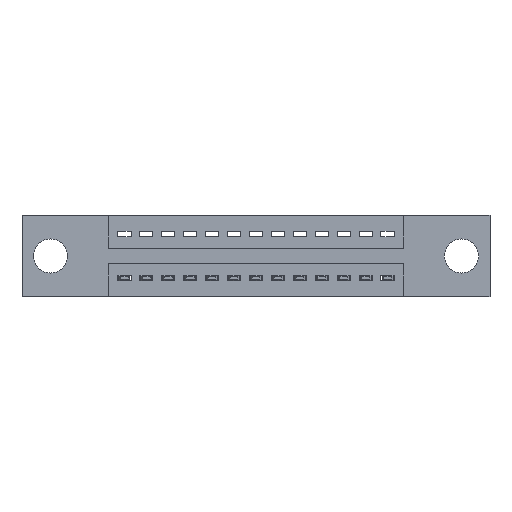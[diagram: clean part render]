
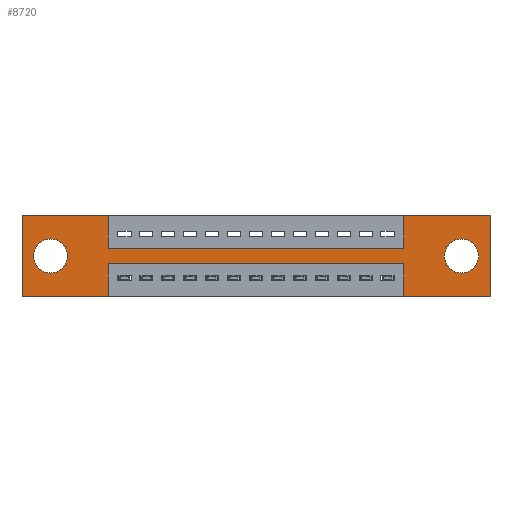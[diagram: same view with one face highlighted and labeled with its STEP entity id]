
A CAD part, front view. The second image highlights one B-rep face of the part: STEP entity #8720.
In plain terms, the highlighted planar face has unit normal (0, -1, 0).
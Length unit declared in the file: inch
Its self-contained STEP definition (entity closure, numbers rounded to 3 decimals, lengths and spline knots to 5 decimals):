
#270 = DIRECTION ( 'NONE',  ( 1., 0., 0. ) ) ;
#277 = VECTOR ( 'NONE', #8580, 39.37008 ) ;
#346 = VERTEX_POINT ( 'NONE', #3894 ) ;
#348 = LINE ( 'NONE', #9882, #1293 ) ;
#350 = CARTESIAN_POINT ( 'NONE',  ( 0.3925, 0., -0.15 ) ) ;
#443 = VERTEX_POINT ( 'NONE', #10243 ) ;
#567 = LINE ( 'NONE', #12195, #5150 ) ;
#646 = VERTEX_POINT ( 'NONE', #5089 ) ;
#901 = CARTESIAN_POINT ( 'NONE',  ( 0.13, 0., -0.107 ) ) ;
#906 = EDGE_CURVE ( 'NONE', #5767, #5690, #348, .T. ) ;
#951 = CARTESIAN_POINT ( 'NONE',  ( 1.7425, 0., -0.37 ) ) ;
#990 = EDGE_CURVE ( 'NONE', #11769, #11636, #4753, .T. ) ;
#1047 = VECTOR ( 'NONE', #12163, 39.37008 ) ;
#1293 = VECTOR ( 'NONE', #1474, 39.37008 ) ;
#1382 = ORIENTED_EDGE ( 'NONE', *, *, #9302, .F. ) ;
#1431 = VERTEX_POINT ( 'NONE', #7428 ) ;
#1454 = VECTOR ( 'NONE', #2695, 39.37008 ) ;
#1474 = DIRECTION ( 'NONE',  ( -1., 0., 0. ) ) ;
#1801 = CARTESIAN_POINT ( 'NONE',  ( 0., 0., -0.37 ) ) ;
#2099 = ORIENTED_EDGE ( 'NONE', *, *, #8531, .T. ) ;
#2127 = ORIENTED_EDGE ( 'NONE', *, *, #5831, .F. ) ;
#2137 = EDGE_CURVE ( 'NONE', #8384, #13415, #567, .T. ) ;
#2385 = FACE_BOUND ( 'NONE', #7747, .T. ) ;
#2518 = LINE ( 'NONE', #8944, #1047 ) ;
#2521 = DIRECTION ( 'NONE',  ( 0., 0., -1. ) ) ;
#2695 = DIRECTION ( 'NONE',  ( 1., 0., 0. ) ) ;
#2714 = VECTOR ( 'NONE', #2521, 39.37008 ) ;
#2877 = LINE ( 'NONE', #9422, #12211 ) ;
#2994 = EDGE_CURVE ( 'NONE', #346, #7902, #2518, .T. ) ;
#3264 = AXIS2_PLACEMENT_3D ( 'NONE', #3440, #4642, #7961 ) ;
#3434 = CARTESIAN_POINT ( 'NONE',  ( 0.3925, 0., 0. ) ) ;
#3440 = CARTESIAN_POINT ( 'NONE',  ( 0., 0., -0.37 ) ) ;
#3488 = ORIENTED_EDGE ( 'NONE', *, *, #11981, .F. ) ;
#3631 = LINE ( 'NONE', #12216, #13633 ) ;
#3663 = VERTEX_POINT ( 'NONE', #12548 ) ;
#3713 = LINE ( 'NONE', #3907, #5990 ) ;
#3721 = CARTESIAN_POINT ( 'NONE',  ( 0.3925, 0., -0.37 ) ) ;
#3894 = CARTESIAN_POINT ( 'NONE',  ( 0., 0., -0.37 ) ) ;
#3907 = CARTESIAN_POINT ( 'NONE',  ( 2.135, 0., 0. ) ) ;
#3952 = AXIS2_PLACEMENT_3D ( 'NONE', #13821, #10790, #12832 ) ;
#4342 = EDGE_CURVE ( 'NONE', #8558, #443, #12095, .T. ) ;
#4457 = CARTESIAN_POINT ( 'NONE',  ( 0., 0., 0. ) ) ;
#4642 = DIRECTION ( 'NONE',  ( 0., -1., 0. ) ) ;
#4753 = CIRCLE ( 'NONE', #10372, 0.078 ) ;
#4829 = CARTESIAN_POINT ( 'NONE',  ( 2.005, 0., -0.185 ) ) ;
#4844 = ORIENTED_EDGE ( 'NONE', *, *, #7290, .F. ) ;
#4914 = ORIENTED_EDGE ( 'NONE', *, *, #990, .T. ) ;
#4940 = CARTESIAN_POINT ( 'NONE',  ( 0.13, 0., -0.185 ) ) ;
#5089 = CARTESIAN_POINT ( 'NONE',  ( 1.7425, 0., -0.22 ) ) ;
#5150 = VECTOR ( 'NONE', #8906, 39.37008 ) ;
#5632 = FACE_OUTER_BOUND ( 'NONE', #6299, .T. ) ;
#5690 = VERTEX_POINT ( 'NONE', #6253 ) ;
#5699 = EDGE_CURVE ( 'NONE', #3663, #1431, #2877, .T. ) ;
#5767 = VERTEX_POINT ( 'NONE', #12012 ) ;
#5794 = VECTOR ( 'NONE', #8311, 39.37008 ) ;
#5831 = EDGE_CURVE ( 'NONE', #646, #8558, #8516, .T. ) ;
#5882 = ORIENTED_EDGE ( 'NONE', *, *, #12371, .T. ) ;
#5990 = VECTOR ( 'NONE', #8092, 39.37008 ) ;
#5998 = CIRCLE ( 'NONE', #3952, 0.078 ) ;
#6052 = DIRECTION ( 'NONE',  ( -1., 0., 0. ) ) ;
#6253 = CARTESIAN_POINT ( 'NONE',  ( 1.7425, 0., -0.37 ) ) ;
#6299 = EDGE_LOOP ( 'NONE', ( #13230, #2127, #3488, #9588, #1382, #6541, #6807, #11499, #13559, #11309, #10766, #4844 ) ) ;
#6483 = CARTESIAN_POINT ( 'NONE',  ( 0.13, 0., -0.263 ) ) ;
#6541 = ORIENTED_EDGE ( 'NONE', *, *, #5699, .F. ) ;
#6593 = CARTESIAN_POINT ( 'NONE',  ( 0.3925, 0., -0.22 ) ) ;
#6807 = ORIENTED_EDGE ( 'NONE', *, *, #10919, .F. ) ;
#6870 = DIRECTION ( 'NONE',  ( 0., 0., 1. ) ) ;
#6879 = CIRCLE ( 'NONE', #12029, 0.078 ) ;
#6924 = AXIS2_PLACEMENT_3D ( 'NONE', #4829, #11451, #10260 ) ;
#7190 = LINE ( 'NONE', #951, #5794 ) ;
#7290 = EDGE_CURVE ( 'NONE', #443, #346, #8429, .T. ) ;
#7428 = CARTESIAN_POINT ( 'NONE',  ( 2.135, 0., 0. ) ) ;
#7747 = EDGE_LOOP ( 'NONE', ( #5882, #4914 ) ) ;
#7817 = EDGE_LOOP ( 'NONE', ( #9727, #2099 ) ) ;
#7902 = VERTEX_POINT ( 'NONE', #4457 ) ;
#7961 = DIRECTION ( 'NONE',  ( 0., 0., -1. ) ) ;
#8046 = VECTOR ( 'NONE', #270, 39.37008 ) ;
#8092 = DIRECTION ( 'NONE',  ( 0., 0., -1. ) ) ;
#8311 = DIRECTION ( 'NONE',  ( 0., 0., 1. ) ) ;
#8384 = VERTEX_POINT ( 'NONE', #3434 ) ;
#8429 = LINE ( 'NONE', #1801, #9529 ) ;
#8516 = LINE ( 'NONE', #6593, #277 ) ;
#8531 = EDGE_CURVE ( 'NONE', #11574, #11751, #6879, .T. ) ;
#8558 = VERTEX_POINT ( 'NONE', #10659 ) ;
#8580 = DIRECTION ( 'NONE',  ( -1., 0., 0. ) ) ;
#8720 = ADVANCED_FACE ( 'NONE', ( #8812, #2385, #5632 ), #11196, .T. ) ;
#8746 = CARTESIAN_POINT ( 'NONE',  ( 2.005, 0., -0.107 ) ) ;
#8812 = FACE_BOUND ( 'NONE', #7817, .T. ) ;
#8906 = DIRECTION ( 'NONE',  ( 0., 0., -1. ) ) ;
#8944 = CARTESIAN_POINT ( 'NONE',  ( 0., 0., 0. ) ) ;
#9139 = VERTEX_POINT ( 'NONE', #11941 ) ;
#9302 = EDGE_CURVE ( 'NONE', #1431, #5767, #3713, .T. ) ;
#9422 = CARTESIAN_POINT ( 'NONE',  ( 0., 0., 0. ) ) ;
#9529 = VECTOR ( 'NONE', #6052, 39.37008 ) ;
#9588 = ORIENTED_EDGE ( 'NONE', *, *, #906, .F. ) ;
#9659 = CARTESIAN_POINT ( 'NONE',  ( 2.005, 0., -0.263 ) ) ;
#9727 = ORIENTED_EDGE ( 'NONE', *, *, #11652, .T. ) ;
#9882 = CARTESIAN_POINT ( 'NONE',  ( 0., 0., -0.37 ) ) ;
#10157 = EDGE_CURVE ( 'NONE', #13415, #9139, #13468, .T. ) ;
#10243 = CARTESIAN_POINT ( 'NONE',  ( 0.3925, 0., -0.37 ) ) ;
#10260 = DIRECTION ( 'NONE',  ( 0., 0., -1. ) ) ;
#10372 = AXIS2_PLACEMENT_3D ( 'NONE', #4940, #13532, #13597 ) ;
#10593 = DIRECTION ( 'NONE',  ( 0., 1., 0. ) ) ;
#10659 = CARTESIAN_POINT ( 'NONE',  ( 0.3925, 0., -0.22 ) ) ;
#10766 = ORIENTED_EDGE ( 'NONE', *, *, #2994, .F. ) ;
#10790 = DIRECTION ( 'NONE',  ( 0., 1., 0. ) ) ;
#10919 = EDGE_CURVE ( 'NONE', #9139, #3663, #3631, .T. ) ;
#11196 = PLANE ( 'NONE',  #3264 ) ;
#11309 = ORIENTED_EDGE ( 'NONE', *, *, #11717, .F. ) ;
#11451 = DIRECTION ( 'NONE',  ( 0., 1., 0. ) ) ;
#11499 = ORIENTED_EDGE ( 'NONE', *, *, #10157, .F. ) ;
#11574 = VERTEX_POINT ( 'NONE', #9659 ) ;
#11636 = VERTEX_POINT ( 'NONE', #901 ) ;
#11652 = EDGE_CURVE ( 'NONE', #11751, #11574, #13882, .T. ) ;
#11717 = EDGE_CURVE ( 'NONE', #7902, #8384, #13026, .T. ) ;
#11751 = VERTEX_POINT ( 'NONE', #8746 ) ;
#11769 = VERTEX_POINT ( 'NONE', #6483 ) ;
#11823 = CARTESIAN_POINT ( 'NONE',  ( 0., 0., 0. ) ) ;
#11941 = CARTESIAN_POINT ( 'NONE',  ( 1.7425, 0., -0.15 ) ) ;
#11958 = CARTESIAN_POINT ( 'NONE',  ( 0.3925, 0., -0.15 ) ) ;
#11981 = EDGE_CURVE ( 'NONE', #5690, #646, #7190, .T. ) ;
#12012 = CARTESIAN_POINT ( 'NONE',  ( 2.135, 0., -0.37 ) ) ;
#12029 = AXIS2_PLACEMENT_3D ( 'NONE', #12699, #10593, #13831 ) ;
#12095 = LINE ( 'NONE', #3721, #2714 ) ;
#12163 = DIRECTION ( 'NONE',  ( 0., 0., 1. ) ) ;
#12195 = CARTESIAN_POINT ( 'NONE',  ( 0.3925, 0., 0. ) ) ;
#12211 = VECTOR ( 'NONE', #12723, 39.37008 ) ;
#12216 = CARTESIAN_POINT ( 'NONE',  ( 1.7425, 0., 0. ) ) ;
#12371 = EDGE_CURVE ( 'NONE', #11636, #11769, #5998, .T. ) ;
#12548 = CARTESIAN_POINT ( 'NONE',  ( 1.7425, 0., 0. ) ) ;
#12699 = CARTESIAN_POINT ( 'NONE',  ( 2.005, 0., -0.185 ) ) ;
#12723 = DIRECTION ( 'NONE',  ( 1., 0., 0. ) ) ;
#12832 = DIRECTION ( 'NONE',  ( 0., 0., 1. ) ) ;
#13026 = LINE ( 'NONE', #11823, #8046 ) ;
#13230 = ORIENTED_EDGE ( 'NONE', *, *, #4342, .F. ) ;
#13415 = VERTEX_POINT ( 'NONE', #11958 ) ;
#13468 = LINE ( 'NONE', #350, #1454 ) ;
#13532 = DIRECTION ( 'NONE',  ( 0., 1., 0. ) ) ;
#13559 = ORIENTED_EDGE ( 'NONE', *, *, #2137, .F. ) ;
#13597 = DIRECTION ( 'NONE',  ( 0., 0., 1. ) ) ;
#13633 = VECTOR ( 'NONE', #6870, 39.37008 ) ;
#13821 = CARTESIAN_POINT ( 'NONE',  ( 0.13, 0., -0.185 ) ) ;
#13831 = DIRECTION ( 'NONE',  ( 0., 0., -1. ) ) ;
#13882 = CIRCLE ( 'NONE', #6924, 0.078 ) ;
